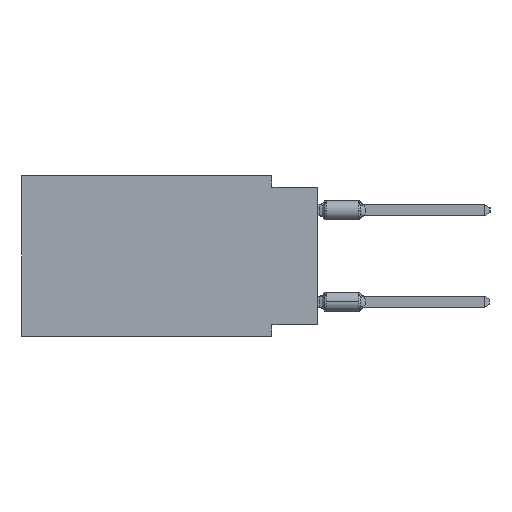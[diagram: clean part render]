
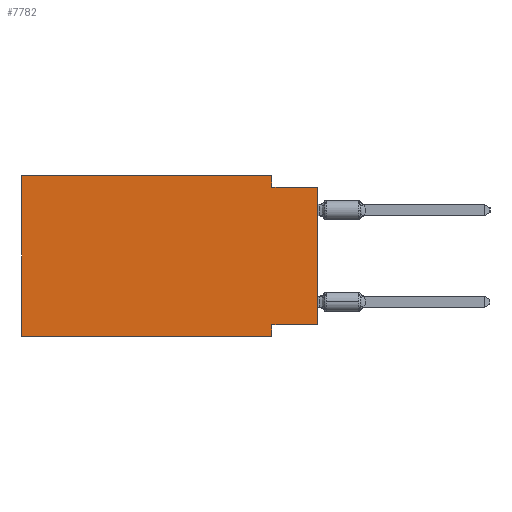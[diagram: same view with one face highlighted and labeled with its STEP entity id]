
A CAD part, left-side view. The second image highlights one B-rep face of the part: STEP entity #7782.
In plain terms, the highlighted planar face has unit normal (-1, 0, 0).
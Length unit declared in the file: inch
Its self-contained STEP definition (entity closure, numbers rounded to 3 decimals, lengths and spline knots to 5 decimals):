
#1876 = EDGE_CURVE ( 'NONE', #7202, #17631, #6255, .T. ) ;
#2030 = ORIENTED_EDGE ( 'NONE', *, *, #23129, .T. ) ;
#2950 = CARTESIAN_POINT ( 'NONE',  ( 0., 0.1, -0.025 ) ) ;
#2953 = EDGE_CURVE ( 'NONE', #17631, #25567, #36727, .T. ) ;
#3141 = LINE ( 'NONE', #26185, #10200 ) ;
#3168 = VERTEX_POINT ( 'NONE', #2950 ) ;
#6255 = LINE ( 'NONE', #17767, #8641 ) ;
#6434 = ORIENTED_EDGE ( 'NONE', *, *, #1876, .F. ) ;
#7202 = VERTEX_POINT ( 'NONE', #20253 ) ;
#7290 = CARTESIAN_POINT ( 'NONE',  ( 0., 0.1, -0.325 ) ) ;
#7335 = DIRECTION ( 'NONE',  ( 0., 0., -1. ) ) ;
#7782 = ADVANCED_FACE ( 'NONE', ( #36019 ), #9616, .F. ) ;
#8416 = LINE ( 'NONE', #11249, #13736 ) ;
#8470 = ORIENTED_EDGE ( 'NONE', *, *, #24624, .F. ) ;
#8633 = DIRECTION ( 'NONE',  ( 0., 1., 0. ) ) ;
#8641 = VECTOR ( 'NONE', #29274, 39.37008 ) ;
#9616 = PLANE ( 'NONE',  #13030 ) ;
#9807 = CARTESIAN_POINT ( 'NONE',  ( 0., 0., -0.025 ) ) ;
#10113 = VECTOR ( 'NONE', #35016, 39.37008 ) ;
#10177 = LINE ( 'NONE', #9807, #20328 ) ;
#10200 = VECTOR ( 'NONE', #8633, 39.37008 ) ;
#10693 = CARTESIAN_POINT ( 'NONE',  ( 0., 0.1, 0. ) ) ;
#10885 = DIRECTION ( 'NONE',  ( 0., 0., -1. ) ) ;
#11249 = CARTESIAN_POINT ( 'NONE',  ( 0., 0.1, -0.35 ) ) ;
#12397 = ORIENTED_EDGE ( 'NONE', *, *, #23970, .F. ) ;
#13030 = AXIS2_PLACEMENT_3D ( 'NONE', #32648, #20951, #7335 ) ;
#13736 = VECTOR ( 'NONE', #22948, 39.37008 ) ;
#13905 = CARTESIAN_POINT ( 'NONE',  ( 0., 0.645, 0. ) ) ;
#13906 = DIRECTION ( 'NONE',  ( 0., 0., 1. ) ) ;
#13977 = VECTOR ( 'NONE', #33528, 39.37008 ) ;
#14711 = VERTEX_POINT ( 'NONE', #16397 ) ;
#15552 = ORIENTED_EDGE ( 'NONE', *, *, #2953, .F. ) ;
#16397 = CARTESIAN_POINT ( 'NONE',  ( 0., 0., -0.025 ) ) ;
#17119 = ORIENTED_EDGE ( 'NONE', *, *, #21352, .T. ) ;
#17234 = VERTEX_POINT ( 'NONE', #7290 ) ;
#17631 = VERTEX_POINT ( 'NONE', #33291 ) ;
#17767 = CARTESIAN_POINT ( 'NONE',  ( 0., 0.645, 0. ) ) ;
#17940 = CARTESIAN_POINT ( 'NONE',  ( 0., 0.1, 0. ) ) ;
#18379 = VERTEX_POINT ( 'NONE', #34611 ) ;
#19690 = VECTOR ( 'NONE', #10885, 39.37008 ) ;
#20253 = CARTESIAN_POINT ( 'NONE',  ( 0., 0.645, -0.35 ) ) ;
#20328 = VECTOR ( 'NONE', #27348, 39.37008 ) ;
#20744 = EDGE_LOOP ( 'NONE', ( #2030, #12397, #30221, #15552, #6434, #17119, #8470, #23944 ) ) ;
#20951 = DIRECTION ( 'NONE',  ( 1., 0., 0. ) ) ;
#21352 = EDGE_CURVE ( 'NONE', #7202, #28261, #23518, .T. ) ;
#22213 = CARTESIAN_POINT ( 'NONE',  ( 0., 0., 0. ) ) ;
#22948 = DIRECTION ( 'NONE',  ( 0., 0., -1. ) ) ;
#23060 = EDGE_CURVE ( 'NONE', #25567, #3168, #28048, .T. ) ;
#23129 = EDGE_CURVE ( 'NONE', #18379, #14711, #25236, .T. ) ;
#23518 = LINE ( 'NONE', #26538, #10113 ) ;
#23944 = ORIENTED_EDGE ( 'NONE', *, *, #37039, .F. ) ;
#23970 = EDGE_CURVE ( 'NONE', #3168, #14711, #10177, .T. ) ;
#24523 = VECTOR ( 'NONE', #13906, 39.37008 ) ;
#24624 = EDGE_CURVE ( 'NONE', #17234, #28261, #8416, .T. ) ;
#25236 = LINE ( 'NONE', #22213, #24523 ) ;
#25567 = VERTEX_POINT ( 'NONE', #17940 ) ;
#26185 = CARTESIAN_POINT ( 'NONE',  ( 0., 0., -0.325 ) ) ;
#26538 = CARTESIAN_POINT ( 'NONE',  ( 0., 0.645, -0.35 ) ) ;
#27348 = DIRECTION ( 'NONE',  ( 0., -1., 0. ) ) ;
#28048 = LINE ( 'NONE', #10693, #19690 ) ;
#28261 = VERTEX_POINT ( 'NONE', #36829 ) ;
#29274 = DIRECTION ( 'NONE',  ( 0., 0., 1. ) ) ;
#30221 = ORIENTED_EDGE ( 'NONE', *, *, #23060, .F. ) ;
#32648 = CARTESIAN_POINT ( 'NONE',  ( 0., 0.645, 0. ) ) ;
#33291 = CARTESIAN_POINT ( 'NONE',  ( 0., 0.645, 0. ) ) ;
#33528 = DIRECTION ( 'NONE',  ( 0., -1., 0. ) ) ;
#34611 = CARTESIAN_POINT ( 'NONE',  ( 0., 0., -0.325 ) ) ;
#35016 = DIRECTION ( 'NONE',  ( 0., -1., 0. ) ) ;
#36019 = FACE_OUTER_BOUND ( 'NONE', #20744, .T. ) ;
#36727 = LINE ( 'NONE', #13905, #13977 ) ;
#36829 = CARTESIAN_POINT ( 'NONE',  ( 0., 0.1, -0.35 ) ) ;
#37039 = EDGE_CURVE ( 'NONE', #18379, #17234, #3141, .T. ) ;
